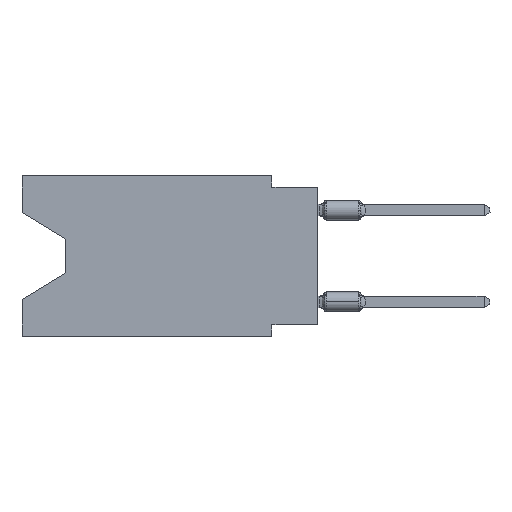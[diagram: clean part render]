
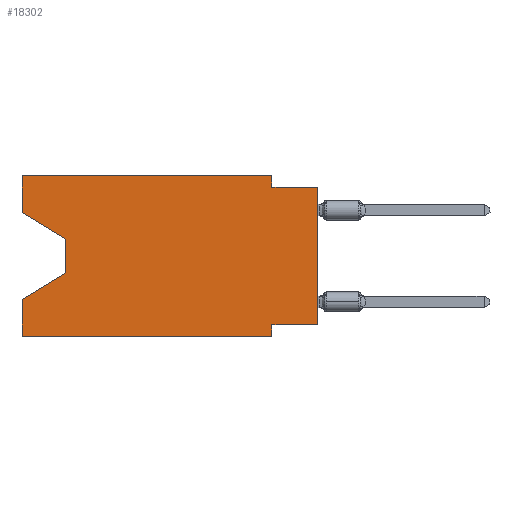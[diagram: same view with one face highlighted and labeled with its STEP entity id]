
A CAD part, left-side view. The second image highlights one B-rep face of the part: STEP entity #18302.
In plain terms, the highlighted planar face has unit normal (-1, 0, 0).
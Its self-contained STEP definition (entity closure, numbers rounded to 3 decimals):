
#157 = CARTESIAN_POINT ( 'NONE',  ( 0., 16.383, -2.038 ) ) ;
#472 = ORIENTED_EDGE ( 'NONE', *, *, #17015, .T. ) ;
#719 = EDGE_CURVE ( 'NONE', #15088, #13613, #13182, .T. ) ;
#907 = LINE ( 'NONE', #15970, #1907 ) ;
#1188 = VERTEX_POINT ( 'NONE', #2414 ) ;
#1750 = VECTOR ( 'NONE', #18474, 1000. ) ;
#1907 = VECTOR ( 'NONE', #21004, 1000. ) ;
#1951 = ORIENTED_EDGE ( 'NONE', *, *, #2596, .F. ) ;
#2414 = CARTESIAN_POINT ( 'NONE',  ( 0., 0., -8.255 ) ) ;
#2596 = EDGE_CURVE ( 'NONE', #9952, #29563, #3059, .T. ) ;
#2899 = DIRECTION ( 'NONE',  ( 0., 0., 1. ) ) ;
#2935 = CARTESIAN_POINT ( 'NONE',  ( 0., 13.97, -3.505 ) ) ;
#2944 = CARTESIAN_POINT ( 'NONE',  ( 0., 2.54, 0. ) ) ;
#3059 = LINE ( 'NONE', #10811, #28362 ) ;
#3111 = DIRECTION ( 'NONE',  ( 0., 0., -1. ) ) ;
#3650 = VECTOR ( 'NONE', #27099, 1000. ) ;
#3766 = CARTESIAN_POINT ( 'NONE',  ( 0., 0., 0. ) ) ;
#3882 = DIRECTION ( 'NONE',  ( 0., 0., -1. ) ) ;
#3896 = VERTEX_POINT ( 'NONE', #5064 ) ;
#5064 = CARTESIAN_POINT ( 'NONE',  ( 0., 2.54, -0.635 ) ) ;
#5200 = CARTESIAN_POINT ( 'NONE',  ( 0., 2.54, -8.255 ) ) ;
#5738 = DIRECTION ( 'NONE',  ( 0., -1., 0. ) ) ;
#6420 = VERTEX_POINT ( 'NONE', #5200 ) ;
#6497 = VECTOR ( 'NONE', #5738, 1000. ) ;
#6672 = CARTESIAN_POINT ( 'NONE',  ( 0., 16.383, -8.89 ) ) ;
#6733 = LINE ( 'NONE', #16467, #1750 ) ;
#7594 = VERTEX_POINT ( 'NONE', #2935 ) ;
#7599 = EDGE_LOOP ( 'NONE', ( #472, #30193, #24993, #1951, #18943, #29032, #19446, #10486, #13718, #24163, #12000, #20817 ) ) ;
#8545 = VECTOR ( 'NONE', #24643, 1000. ) ;
#8553 = VERTEX_POINT ( 'NONE', #9256 ) ;
#8725 = EDGE_CURVE ( 'NONE', #32055, #15088, #24357, .T. ) ;
#9256 = CARTESIAN_POINT ( 'NONE',  ( 0., 13.97, -5.385 ) ) ;
#9332 = VECTOR ( 'NONE', #14287, 1000. ) ;
#9653 = AXIS2_PLACEMENT_3D ( 'NONE', #16037, #13753, #3882 ) ;
#9952 = VERTEX_POINT ( 'NONE', #29373 ) ;
#10260 = LINE ( 'NONE', #23254, #17282 ) ;
#10486 = ORIENTED_EDGE ( 'NONE', *, *, #17913, .T. ) ;
#10811 = CARTESIAN_POINT ( 'NONE',  ( 0., 16.383, 0. ) ) ;
#11723 = VECTOR ( 'NONE', #25855, 1000. ) ;
#12000 = ORIENTED_EDGE ( 'NONE', *, *, #719, .F. ) ;
#12149 = EDGE_CURVE ( 'NONE', #1188, #6420, #27989, .T. ) ;
#13074 = EDGE_CURVE ( 'NONE', #3896, #25435, #10260, .T. ) ;
#13182 = LINE ( 'NONE', #27957, #6497 ) ;
#13196 = CARTESIAN_POINT ( 'NONE',  ( 0., 2.54, -8.89 ) ) ;
#13207 = DIRECTION ( 'NONE',  ( 0., 1., 0. ) ) ;
#13613 = VERTEX_POINT ( 'NONE', #31166 ) ;
#13718 = ORIENTED_EDGE ( 'NONE', *, *, #13074, .F. ) ;
#13753 = DIRECTION ( 'NONE',  ( 1., 0., 0. ) ) ;
#14005 = EDGE_CURVE ( 'NONE', #7594, #8553, #6733, .T. ) ;
#14287 = DIRECTION ( 'NONE',  ( 0., -1., 0. ) ) ;
#14746 = LINE ( 'NONE', #157, #8545 ) ;
#15088 = VERTEX_POINT ( 'NONE', #19946 ) ;
#15970 = CARTESIAN_POINT ( 'NONE',  ( 0., 13.97, -5.385 ) ) ;
#16037 = CARTESIAN_POINT ( 'NONE',  ( 0., 16.383, 0. ) ) ;
#16467 = CARTESIAN_POINT ( 'NONE',  ( 0., 13.97, -3.505 ) ) ;
#16593 = CARTESIAN_POINT ( 'NONE',  ( 0., 16.383, -6.852 ) ) ;
#17015 = EDGE_CURVE ( 'NONE', #32055, #7594, #14746, .T. ) ;
#17282 = VECTOR ( 'NONE', #25365, 1000. ) ;
#17508 = FACE_OUTER_BOUND ( 'NONE', #7599, .T. ) ;
#17684 = LINE ( 'NONE', #2944, #20811 ) ;
#17913 = EDGE_CURVE ( 'NONE', #1188, #25435, #18519, .T. ) ;
#17983 = VERTEX_POINT ( 'NONE', #26118 ) ;
#18302 = ADVANCED_FACE ( 'NONE', ( #17508 ), #28527, .F. ) ;
#18474 = DIRECTION ( 'NONE',  ( 0., 0., -1. ) ) ;
#18519 = LINE ( 'NONE', #3766, #26723 ) ;
#18943 = ORIENTED_EDGE ( 'NONE', *, *, #24462, .T. ) ;
#18998 = LINE ( 'NONE', #6672, #9332 ) ;
#19161 = EDGE_CURVE ( 'NONE', #6420, #17983, #30741, .T. ) ;
#19446 = ORIENTED_EDGE ( 'NONE', *, *, #12149, .F. ) ;
#19946 = CARTESIAN_POINT ( 'NONE',  ( 0., 16.383, 0. ) ) ;
#20450 = EDGE_CURVE ( 'NONE', #8553, #29563, #907, .T. ) ;
#20684 = CARTESIAN_POINT ( 'NONE',  ( 0., 0., -8.255 ) ) ;
#20811 = VECTOR ( 'NONE', #3111, 1000. ) ;
#20817 = ORIENTED_EDGE ( 'NONE', *, *, #8725, .F. ) ;
#21004 = DIRECTION ( 'NONE',  ( 0., 0.855, -0.519 ) ) ;
#22401 = VECTOR ( 'NONE', #13207, 1000. ) ;
#22588 = CARTESIAN_POINT ( 'NONE',  ( 0., 0., -0.635 ) ) ;
#22624 = CARTESIAN_POINT ( 'NONE',  ( 0., 16.383, -2.038 ) ) ;
#23254 = CARTESIAN_POINT ( 'NONE',  ( 0., 0., -0.635 ) ) ;
#24163 = ORIENTED_EDGE ( 'NONE', *, *, #25986, .F. ) ;
#24357 = LINE ( 'NONE', #29707, #3650 ) ;
#24462 = EDGE_CURVE ( 'NONE', #9952, #17983, #18998, .T. ) ;
#24643 = DIRECTION ( 'NONE',  ( 0., -0.855, -0.519 ) ) ;
#24993 = ORIENTED_EDGE ( 'NONE', *, *, #20450, .T. ) ;
#25365 = DIRECTION ( 'NONE',  ( 0., -1., 0. ) ) ;
#25435 = VERTEX_POINT ( 'NONE', #22588 ) ;
#25651 = DIRECTION ( 'NONE',  ( 0., 0., 1. ) ) ;
#25855 = DIRECTION ( 'NONE',  ( 0., 0., -1. ) ) ;
#25986 = EDGE_CURVE ( 'NONE', #13613, #3896, #17684, .T. ) ;
#26118 = CARTESIAN_POINT ( 'NONE',  ( 0., 2.54, -8.89 ) ) ;
#26723 = VECTOR ( 'NONE', #25651, 1000. ) ;
#27099 = DIRECTION ( 'NONE',  ( 0., 0., 1. ) ) ;
#27957 = CARTESIAN_POINT ( 'NONE',  ( 0., 16.383, 0. ) ) ;
#27989 = LINE ( 'NONE', #20684, #22401 ) ;
#28362 = VECTOR ( 'NONE', #2899, 1000. ) ;
#28527 = PLANE ( 'NONE',  #9653 ) ;
#29032 = ORIENTED_EDGE ( 'NONE', *, *, #19161, .F. ) ;
#29373 = CARTESIAN_POINT ( 'NONE',  ( 0., 16.383, -8.89 ) ) ;
#29563 = VERTEX_POINT ( 'NONE', #16593 ) ;
#29707 = CARTESIAN_POINT ( 'NONE',  ( 0., 16.383, 0. ) ) ;
#30193 = ORIENTED_EDGE ( 'NONE', *, *, #14005, .T. ) ;
#30741 = LINE ( 'NONE', #13196, #11723 ) ;
#31166 = CARTESIAN_POINT ( 'NONE',  ( 0., 2.54, 0. ) ) ;
#32055 = VERTEX_POINT ( 'NONE', #22624 ) ;
